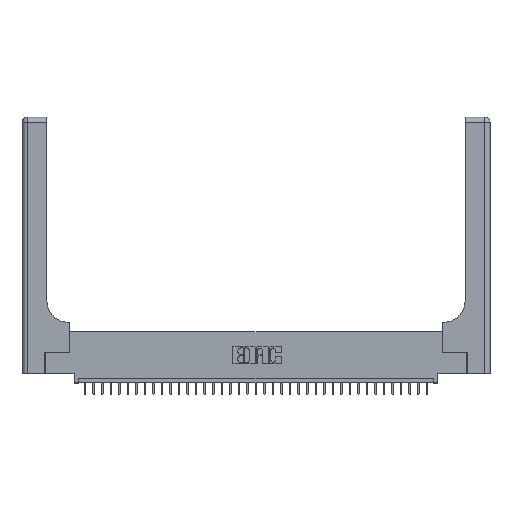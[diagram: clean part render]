
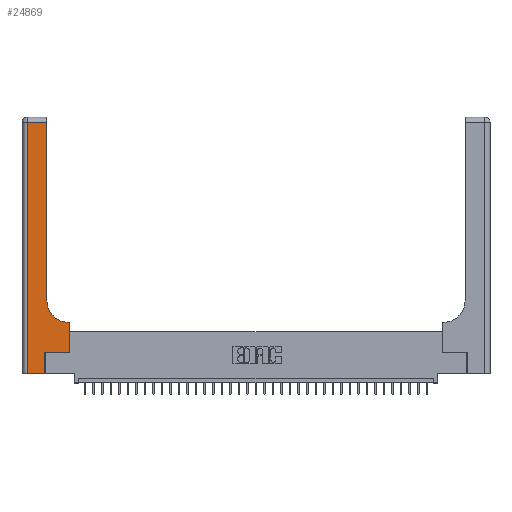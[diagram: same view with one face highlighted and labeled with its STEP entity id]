
A CAD part, top view. The second image highlights one B-rep face of the part: STEP entity #24869.
In plain terms, the highlighted planar face has unit normal (0, 0, 1).
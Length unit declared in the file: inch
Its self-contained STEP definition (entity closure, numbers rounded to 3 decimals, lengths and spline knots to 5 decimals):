
#51 = PLANE ( 'NONE',  #7703 ) ;
#195 = EDGE_CURVE ( 'NONE', #23533, #34035, #13497, .T. ) ;
#834 = CARTESIAN_POINT ( 'NONE',  ( 0.5585, 0.25, 0.37 ) ) ;
#1105 = VECTOR ( 'NONE', #16460, 39.37008 ) ;
#1252 = LINE ( 'NONE', #32755, #2639 ) ;
#2173 = ORIENTED_EDGE ( 'NONE', *, *, #34391, .T. ) ;
#2639 = VECTOR ( 'NONE', #7129, 39.37008 ) ;
#2935 = LINE ( 'NONE', #10886, #31109 ) ;
#2994 = VECTOR ( 'NONE', #5188, 39.37008 ) ;
#3125 = EDGE_LOOP ( 'NONE', ( #11663, #18886, #2173, #16546, #17676, #29833, #9535, #12242, #32550 ) ) ;
#3650 = VERTEX_POINT ( 'NONE', #14505 ) ;
#5188 = DIRECTION ( 'NONE',  ( 0., 1., 0. ) ) ;
#6167 = EDGE_CURVE ( 'NONE', #3650, #8793, #34990, .T. ) ;
#7129 = DIRECTION ( 'NONE',  ( -1., 0., 0. ) ) ;
#7609 = VERTEX_POINT ( 'NONE', #29974 ) ;
#7703 = AXIS2_PLACEMENT_3D ( 'NONE', #10727, #27876, #10912 ) ;
#7949 = LINE ( 'NONE', #27885, #1105 ) ;
#8130 = CARTESIAN_POINT ( 'NONE',  ( 0.2915, 3., 0.37 ) ) ;
#8692 = VERTEX_POINT ( 'NONE', #22807 ) ;
#8793 = VERTEX_POINT ( 'NONE', #25758 ) ;
#9232 = EDGE_CURVE ( 'NONE', #7609, #8692, #31427, .T. ) ;
#9535 = ORIENTED_EDGE ( 'NONE', *, *, #9232, .T. ) ;
#9782 = DIRECTION ( 'NONE',  ( 0., 1., 0. ) ) ;
#10727 = CARTESIAN_POINT ( 'NONE',  ( 0., 3., 0.37 ) ) ;
#10886 = CARTESIAN_POINT ( 'NONE',  ( 0., 2.94, 0.37 ) ) ;
#10912 = DIRECTION ( 'NONE',  ( -1., 0., 0. ) ) ;
#11174 = VERTEX_POINT ( 'NONE', #29971 ) ;
#11586 = EDGE_CURVE ( 'NONE', #11174, #7609, #35259, .T. ) ;
#11663 = ORIENTED_EDGE ( 'NONE', *, *, #195, .T. ) ;
#12242 = ORIENTED_EDGE ( 'NONE', *, *, #15581, .T. ) ;
#12564 = LINE ( 'NONE', #23805, #29540 ) ;
#13496 = FACE_OUTER_BOUND ( 'NONE', #3125, .T. ) ;
#13497 = LINE ( 'NONE', #8130, #2994 ) ;
#14505 = CARTESIAN_POINT ( 'NONE',  ( 0.06, 0., 0.37 ) ) ;
#15024 = DIRECTION ( 'NONE',  ( 0., 1., 0. ) ) ;
#15193 = DIRECTION ( 'NONE',  ( 1., 0., 0. ) ) ;
#15581 = EDGE_CURVE ( 'NONE', #8692, #31474, #1252, .T. ) ;
#16460 = DIRECTION ( 'NONE',  ( 0., -1., 0. ) ) ;
#16546 = ORIENTED_EDGE ( 'NONE', *, *, #6167, .T. ) ;
#16566 = VECTOR ( 'NONE', #15024, 39.37008 ) ;
#17676 = ORIENTED_EDGE ( 'NONE', *, *, #25885, .T. ) ;
#17870 = VECTOR ( 'NONE', #15193, 39.37008 ) ;
#18111 = CARTESIAN_POINT ( 'NONE',  ( 0.2915, 0.85, 0.37 ) ) ;
#18483 = VERTEX_POINT ( 'NONE', #33666 ) ;
#18886 = ORIENTED_EDGE ( 'NONE', *, *, #20709, .T. ) ;
#20709 = EDGE_CURVE ( 'NONE', #34035, #18483, #2935, .T. ) ;
#22314 = DIRECTION ( 'NONE',  ( -1., 0., 0. ) ) ;
#22541 = EDGE_CURVE ( 'NONE', #31474, #23533, #35252, .T. ) ;
#22745 = CARTESIAN_POINT ( 'NONE',  ( 0.2915, 2.94, 0.37 ) ) ;
#22807 = CARTESIAN_POINT ( 'NONE',  ( 0.5585, 0.6, 0.37 ) ) ;
#23533 = VERTEX_POINT ( 'NONE', #18111 ) ;
#23805 = CARTESIAN_POINT ( 'NONE',  ( 0.269, 0., 0.37 ) ) ;
#24745 = VECTOR ( 'NONE', #32593, 39.37008 ) ;
#24869 = ADVANCED_FACE ( 'NONE', ( #13496 ), #51, .F. ) ;
#24918 = DIRECTION ( 'NONE',  ( 1., 0., 0. ) ) ;
#25758 = CARTESIAN_POINT ( 'NONE',  ( 0.269, 0., 0.37 ) ) ;
#25885 = EDGE_CURVE ( 'NONE', #8793, #11174, #12564, .T. ) ;
#27627 = AXIS2_PLACEMENT_3D ( 'NONE', #27865, #33014, #24918 ) ;
#27865 = CARTESIAN_POINT ( 'NONE',  ( 0.5415, 0.85, 0.37 ) ) ;
#27876 = DIRECTION ( 'NONE',  ( 0., 0., -1. ) ) ;
#27885 = CARTESIAN_POINT ( 'NONE',  ( 0.06, 3., 0.37 ) ) ;
#29194 = CARTESIAN_POINT ( 'NONE',  ( 0.269, 0.25, 0.37 ) ) ;
#29540 = VECTOR ( 'NONE', #9782, 39.37008 ) ;
#29833 = ORIENTED_EDGE ( 'NONE', *, *, #11586, .T. ) ;
#29971 = CARTESIAN_POINT ( 'NONE',  ( 0.269, 0.25, 0.37 ) ) ;
#29974 = CARTESIAN_POINT ( 'NONE',  ( 0.5585, 0.25, 0.37 ) ) ;
#31109 = VECTOR ( 'NONE', #22314, 39.37008 ) ;
#31427 = LINE ( 'NONE', #834, #16566 ) ;
#31474 = VERTEX_POINT ( 'NONE', #35879 ) ;
#32550 = ORIENTED_EDGE ( 'NONE', *, *, #22541, .T. ) ;
#32593 = DIRECTION ( 'NONE',  ( 1., 0., 0. ) ) ;
#32755 = CARTESIAN_POINT ( 'NONE',  ( 0.2915, 0.6, 0.37 ) ) ;
#33014 = DIRECTION ( 'NONE',  ( 0., 0., -1. ) ) ;
#33666 = CARTESIAN_POINT ( 'NONE',  ( 0.06, 2.94, 0.37 ) ) ;
#34035 = VERTEX_POINT ( 'NONE', #22745 ) ;
#34391 = EDGE_CURVE ( 'NONE', #18483, #3650, #7949, .T. ) ;
#34990 = LINE ( 'NONE', #35704, #24745 ) ;
#35252 = CIRCLE ( 'NONE', #27627, 0.25 ) ;
#35259 = LINE ( 'NONE', #29194, #17870 ) ;
#35704 = CARTESIAN_POINT ( 'NONE',  ( 0., 0., 0.37 ) ) ;
#35879 = CARTESIAN_POINT ( 'NONE',  ( 0.5415, 0.6, 0.37 ) ) ;
